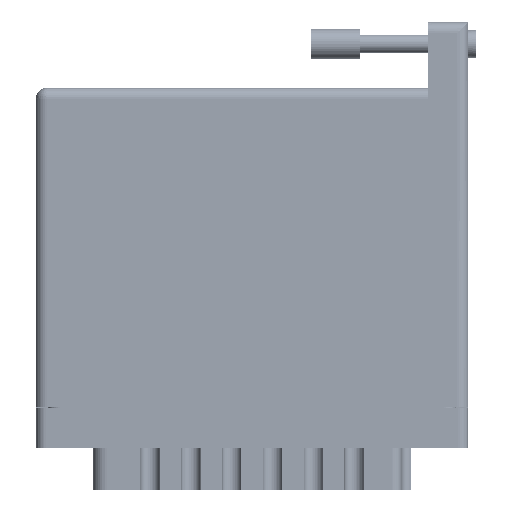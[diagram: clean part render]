
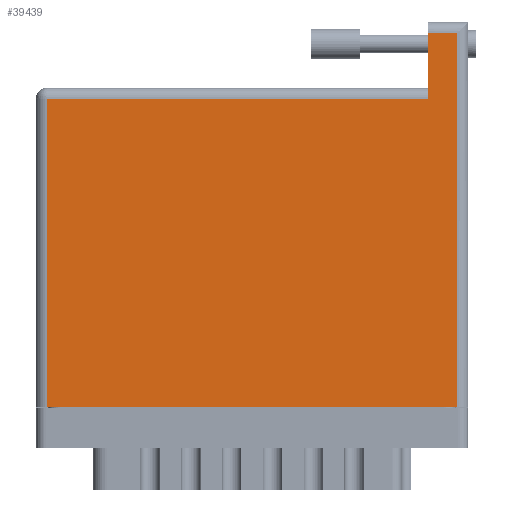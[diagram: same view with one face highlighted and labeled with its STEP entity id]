
A CAD part, front view. The second image highlights one B-rep face of the part: STEP entity #39439.
In plain terms, the highlighted face is planar.
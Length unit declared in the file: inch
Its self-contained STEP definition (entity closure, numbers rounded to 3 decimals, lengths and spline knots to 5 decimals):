
#764 = DIRECTION ( 'NONE',  ( 0., -1., 0. ) ) ;
#6992 = CARTESIAN_POINT ( 'NONE',  ( 0.07, 0., 0. ) ) ;
#8026 = ORIENTED_EDGE ( 'NONE', *, *, #44867, .T. ) ;
#10173 = CARTESIAN_POINT ( 'NONE',  ( 0.07, 0., 0. ) ) ;
#11245 = VECTOR ( 'NONE', #60666, 39.37008 ) ;
#12787 = VERTEX_POINT ( 'NONE', #93287 ) ;
#14863 = CARTESIAN_POINT ( 'NONE',  ( 2.499, 2.45, 0. ) ) ;
#15629 = AXIS2_PLACEMENT_3D ( 'NONE', #68295, #68613, #69581 ) ;
#22642 = ORIENTED_EDGE ( 'NONE', *, *, #91758, .T. ) ;
#22928 = CARTESIAN_POINT ( 'NONE',  ( 0., 0., 0. ) ) ;
#26772 = EDGE_CURVE ( 'NONE', #82823, #52069, #58290, .T. ) ;
#27716 = CARTESIAN_POINT ( 'NONE',  ( 2.685, 2.38, 0. ) ) ;
#27828 = CARTESIAN_POINT ( 'NONE',  ( 2.499, 2.38, 0. ) ) ;
#28196 = CARTESIAN_POINT ( 'NONE',  ( 0.07, 1.96, 0. ) ) ;
#31083 = LINE ( 'NONE', #22928, #11245 ) ;
#32016 = PLANE ( 'NONE',  #15629 ) ;
#32498 = DIRECTION ( 'NONE',  ( -1., 0., 0. ) ) ;
#34946 = VECTOR ( 'NONE', #59759, 39.37008 ) ;
#35340 = LINE ( 'NONE', #38807, #95723 ) ;
#38807 = CARTESIAN_POINT ( 'NONE',  ( 0., 2.38, 0. ) ) ;
#39439 = ADVANCED_FACE ( 'NONE', ( #81930 ), #32016, .F. ) ;
#41195 = EDGE_CURVE ( 'NONE', #12787, #46581, #83007, .T. ) ;
#42519 = CARTESIAN_POINT ( 'NONE',  ( 2.685, 2.45, 0. ) ) ;
#44867 = EDGE_CURVE ( 'NONE', #58811, #12787, #31083, .T. ) ;
#46581 = VERTEX_POINT ( 'NONE', #27716 ) ;
#48448 = VECTOR ( 'NONE', #32498, 39.37008 ) ;
#49112 = ORIENTED_EDGE ( 'NONE', *, *, #41195, .T. ) ;
#52069 = VERTEX_POINT ( 'NONE', #76708 ) ;
#56636 = EDGE_CURVE ( 'NONE', #52069, #57289, #93699, .T. ) ;
#57289 = VERTEX_POINT ( 'NONE', #28196 ) ;
#58290 = LINE ( 'NONE', #14863, #34946 ) ;
#58811 = VERTEX_POINT ( 'NONE', #10173 ) ;
#59759 = DIRECTION ( 'NONE',  ( 0., -1., 0. ) ) ;
#60666 = DIRECTION ( 'NONE',  ( 1., 0., 0. ) ) ;
#60876 = DIRECTION ( 'NONE',  ( -1., 0., 0. ) ) ;
#68295 = CARTESIAN_POINT ( 'NONE',  ( 0., 2.03, 0. ) ) ;
#68613 = DIRECTION ( 'NONE',  ( 0., 0., -1. ) ) ;
#69581 = DIRECTION ( 'NONE',  ( -1., 0., 0. ) ) ;
#76708 = CARTESIAN_POINT ( 'NONE',  ( 2.499, 1.96, 0. ) ) ;
#78123 = EDGE_LOOP ( 'NONE', ( #86056, #94970, #22642, #8026, #49112, #82935 ) ) ;
#81930 = FACE_OUTER_BOUND ( 'NONE', #78123, .T. ) ;
#82280 = LINE ( 'NONE', #6992, #96259 ) ;
#82823 = VERTEX_POINT ( 'NONE', #27828 ) ;
#82935 = ORIENTED_EDGE ( 'NONE', *, *, #88906, .T. ) ;
#83007 = LINE ( 'NONE', #42519, #95779 ) ;
#86056 = ORIENTED_EDGE ( 'NONE', *, *, #26772, .T. ) ;
#88906 = EDGE_CURVE ( 'NONE', #46581, #82823, #35340, .T. ) ;
#91758 = EDGE_CURVE ( 'NONE', #57289, #58811, #82280, .T. ) ;
#91903 = CARTESIAN_POINT ( 'NONE',  ( 0., 1.96, 0. ) ) ;
#93287 = CARTESIAN_POINT ( 'NONE',  ( 2.685, 0., 0. ) ) ;
#93699 = LINE ( 'NONE', #91903, #48448 ) ;
#94970 = ORIENTED_EDGE ( 'NONE', *, *, #56636, .T. ) ;
#95059 = DIRECTION ( 'NONE',  ( 0., 1., 0. ) ) ;
#95723 = VECTOR ( 'NONE', #60876, 39.37008 ) ;
#95779 = VECTOR ( 'NONE', #95059, 39.37008 ) ;
#96259 = VECTOR ( 'NONE', #764, 39.37008 ) ;
